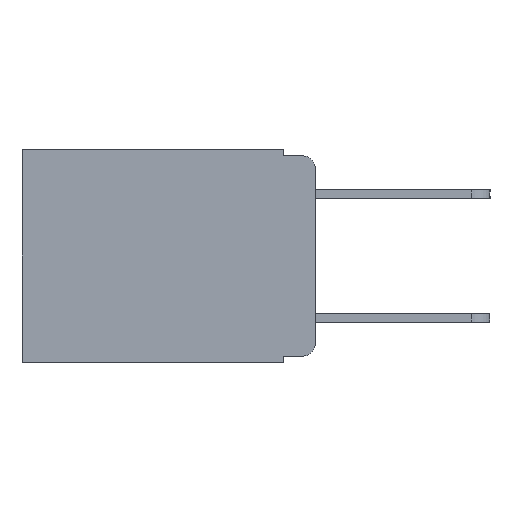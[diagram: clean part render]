
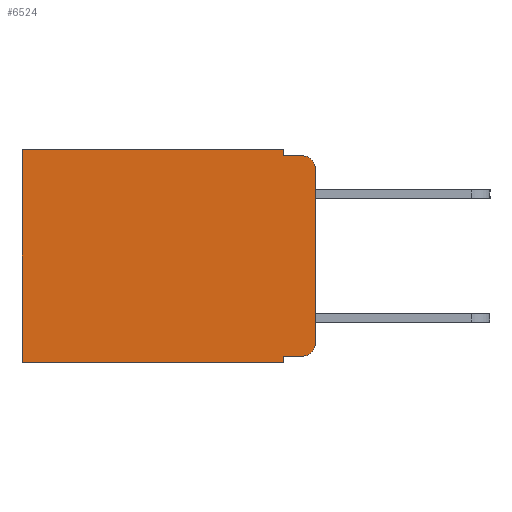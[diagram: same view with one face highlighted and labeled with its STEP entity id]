
A CAD part, left-side view. The second image highlights one B-rep face of the part: STEP entity #6524.
In plain terms, the highlighted planar face has unit normal (-1, 0, 0).
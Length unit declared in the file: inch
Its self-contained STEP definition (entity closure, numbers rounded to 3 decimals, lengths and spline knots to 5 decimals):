
#27 = DIRECTION ( 'NONE',  ( 0., 0., -1. ) ) ;
#486 = VERTEX_POINT ( 'NONE', #5292 ) ;
#596 = CARTESIAN_POINT ( 'NONE',  ( 0.298, 0.051, -0.333 ) ) ;
#648 = CARTESIAN_POINT ( 'NONE',  ( 0.298, 0.02, -0.333 ) ) ;
#745 = CARTESIAN_POINT ( 'NONE',  ( 0.298, 0.051, -0.01 ) ) ;
#789 = VERTEX_POINT ( 'NONE', #6054 ) ;
#850 = EDGE_CURVE ( 'NONE', #15347, #789, #7931, .T. ) ;
#882 = EDGE_CURVE ( 'NONE', #486, #15347, #10780, .T. ) ;
#974 = VERTEX_POINT ( 'NONE', #13333 ) ;
#995 = VERTEX_POINT ( 'NONE', #13096 ) ;
#1546 = EDGE_CURVE ( 'NONE', #9871, #995, #9847, .T. ) ;
#1569 = EDGE_CURVE ( 'NONE', #12250, #11801, #3141, .T. ) ;
#1704 = EDGE_CURVE ( 'NONE', #974, #11801, #15305, .T. ) ;
#1898 = ORIENTED_EDGE ( 'NONE', *, *, #14251, .F. ) ;
#2042 = EDGE_CURVE ( 'NONE', #486, #12250, #12826, .T. ) ;
#2083 = DIRECTION ( 'NONE',  ( 0., 1., 0. ) ) ;
#2128 = DIRECTION ( 'NONE',  ( 0., -1., 0. ) ) ;
#2138 = DIRECTION ( 'NONE',  ( -1., 0., 0. ) ) ;
#2314 = ORIENTED_EDGE ( 'NONE', *, *, #1704, .T. ) ;
#2518 = EDGE_CURVE ( 'NONE', #9577, #3984, #5624, .T. ) ;
#2696 = ORIENTED_EDGE ( 'NONE', *, *, #2042, .F. ) ;
#2734 = VECTOR ( 'NONE', #6627, 39.37008 ) ;
#3141 = LINE ( 'NONE', #5085, #2734 ) ;
#3303 = EDGE_LOOP ( 'NONE', ( #11281, #15026, #1898, #11789, #5516, #2314, #9424, #2696, #9815, #12540 ) ) ;
#3306 = DIRECTION ( 'NONE',  ( 0., 0., -1. ) ) ;
#3984 = VERTEX_POINT ( 'NONE', #12120 ) ;
#4164 = PLANE ( 'NONE',  #6043 ) ;
#5008 = CARTESIAN_POINT ( 'NONE',  ( 0.298, 0.473, 0. ) ) ;
#5034 = CARTESIAN_POINT ( 'NONE',  ( 0.298, 0.473, -0.343 ) ) ;
#5085 = CARTESIAN_POINT ( 'NONE',  ( 0.298, 0., -0.343 ) ) ;
#5275 = FACE_OUTER_BOUND ( 'NONE', #3303, .T. ) ;
#5292 = CARTESIAN_POINT ( 'NONE',  ( 0.298, 0.051, -0.333 ) ) ;
#5300 = LINE ( 'NONE', #745, #14507 ) ;
#5516 = ORIENTED_EDGE ( 'NONE', *, *, #10811, .T. ) ;
#5548 = VECTOR ( 'NONE', #15627, 39.37008 ) ;
#5624 = CIRCLE ( 'NONE', #12181, 0.02 ) ;
#6043 = AXIS2_PLACEMENT_3D ( 'NONE', #15390, #12463, #12537 ) ;
#6054 = CARTESIAN_POINT ( 'NONE',  ( 0.298, 0., -0.313 ) ) ;
#6097 = DIRECTION ( 'NONE',  ( 0., 0., -1. ) ) ;
#6524 = ADVANCED_FACE ( 'NONE', ( #5275 ), #4164, .F. ) ;
#6626 = CARTESIAN_POINT ( 'NONE',  ( 0.298, 0.051, 0. ) ) ;
#6627 = DIRECTION ( 'NONE',  ( 0., 1., 0. ) ) ;
#6783 = DIRECTION ( 'NONE',  ( 0., -1., 0. ) ) ;
#6975 = VECTOR ( 'NONE', #3306, 39.37008 ) ;
#7559 = VECTOR ( 'NONE', #6783, 39.37008 ) ;
#7931 = CIRCLE ( 'NONE', #14372, 0.02 ) ;
#9424 = ORIENTED_EDGE ( 'NONE', *, *, #1569, .F. ) ;
#9577 = VERTEX_POINT ( 'NONE', #9812 ) ;
#9600 = CARTESIAN_POINT ( 'NONE',  ( 0.298, 0.02, -0.313 ) ) ;
#9743 = VECTOR ( 'NONE', #6097, 39.37008 ) ;
#9812 = CARTESIAN_POINT ( 'NONE',  ( 0.298, 0., -0.03 ) ) ;
#9815 = ORIENTED_EDGE ( 'NONE', *, *, #882, .T. ) ;
#9847 = LINE ( 'NONE', #10862, #6975 ) ;
#9871 = VERTEX_POINT ( 'NONE', #10571 ) ;
#10065 = EDGE_CURVE ( 'NONE', #9577, #789, #12014, .T. ) ;
#10184 = DIRECTION ( 'NONE',  ( 0., 0., -1. ) ) ;
#10317 = DIRECTION ( 'NONE',  ( 0., 0., -1. ) ) ;
#10571 = CARTESIAN_POINT ( 'NONE',  ( 0.298, 0.051, 0. ) ) ;
#10780 = LINE ( 'NONE', #596, #7559 ) ;
#10811 = EDGE_CURVE ( 'NONE', #9871, #974, #12837, .T. ) ;
#10862 = CARTESIAN_POINT ( 'NONE',  ( 0.298, 0.051, 0. ) ) ;
#11281 = ORIENTED_EDGE ( 'NONE', *, *, #10065, .F. ) ;
#11739 = VECTOR ( 'NONE', #2083, 39.37008 ) ;
#11789 = ORIENTED_EDGE ( 'NONE', *, *, #1546, .F. ) ;
#11801 = VERTEX_POINT ( 'NONE', #5034 ) ;
#11995 = CARTESIAN_POINT ( 'NONE',  ( 0.298, 0., 0. ) ) ;
#12014 = LINE ( 'NONE', #12219, #5548 ) ;
#12120 = CARTESIAN_POINT ( 'NONE',  ( 0.298, 0.02, -0.01 ) ) ;
#12181 = AXIS2_PLACEMENT_3D ( 'NONE', #13726, #2138, #27 ) ;
#12219 = CARTESIAN_POINT ( 'NONE',  ( 0.298, 0., 0. ) ) ;
#12250 = VERTEX_POINT ( 'NONE', #13231 ) ;
#12289 = VECTOR ( 'NONE', #10317, 39.37008 ) ;
#12463 = DIRECTION ( 'NONE',  ( 1., 0., 0. ) ) ;
#12537 = DIRECTION ( 'NONE',  ( 0., 0., -1. ) ) ;
#12540 = ORIENTED_EDGE ( 'NONE', *, *, #850, .T. ) ;
#12826 = LINE ( 'NONE', #6626, #9743 ) ;
#12837 = LINE ( 'NONE', #11995, #11739 ) ;
#13096 = CARTESIAN_POINT ( 'NONE',  ( 0.298, 0.051, -0.01 ) ) ;
#13231 = CARTESIAN_POINT ( 'NONE',  ( 0.298, 0.051, -0.343 ) ) ;
#13333 = CARTESIAN_POINT ( 'NONE',  ( 0.298, 0.473, 0. ) ) ;
#13726 = CARTESIAN_POINT ( 'NONE',  ( 0.298, 0.02, -0.03 ) ) ;
#14251 = EDGE_CURVE ( 'NONE', #995, #3984, #5300, .T. ) ;
#14372 = AXIS2_PLACEMENT_3D ( 'NONE', #9600, #14550, #10184 ) ;
#14507 = VECTOR ( 'NONE', #2128, 39.37008 ) ;
#14550 = DIRECTION ( 'NONE',  ( -1., 0., 0. ) ) ;
#15026 = ORIENTED_EDGE ( 'NONE', *, *, #2518, .T. ) ;
#15305 = LINE ( 'NONE', #5008, #12289 ) ;
#15347 = VERTEX_POINT ( 'NONE', #648 ) ;
#15390 = CARTESIAN_POINT ( 'NONE',  ( 0.298, 0., 0. ) ) ;
#15627 = DIRECTION ( 'NONE',  ( 0., 0., -1. ) ) ;
